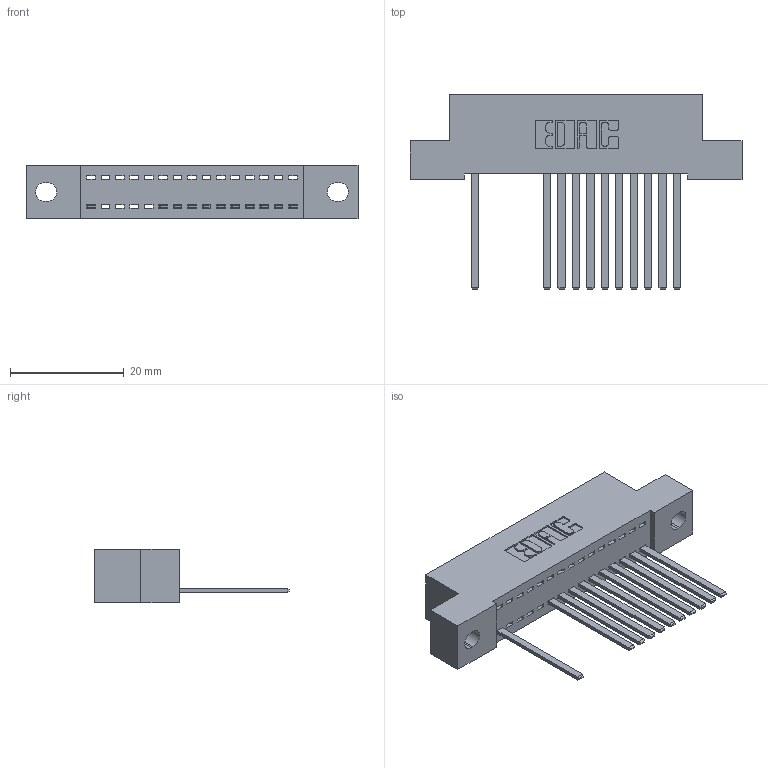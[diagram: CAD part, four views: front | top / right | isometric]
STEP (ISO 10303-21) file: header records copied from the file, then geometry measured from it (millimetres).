
FILE_DESCRIPTION (( 'STEP AP203' ), '1' );
FILE_NAME ('392-015-544-102.STEP', '2018-08-15T01:08:41', ( '' ), ( '' ), 'SwSTEP 2.0', 'SolidWorks 2016', '' );
FILE_SCHEMA (( 'CONFIG_CONTROL_DESIGN' ));
Length unit declared in the file: inch
Products named in the file (3): 342 Part_.128 Slot; 345-292-001_345-293-144; 392-015-544-102
Assembly tree (12 placements, depth 2):
  392-015-544-102
    342 Part_.128 Slot
    345-292-001_345-293-144  x11
Bounding box: 58.42 x 34.3 x 9.4 mm (x, y, z)
Volume: 5052.3 mm3; surface area: 6800.1 mm2
Topology: 12 solids, 12 shells, 734 faces, 2217 edges, 1462 vertices
Faces by surface type: plane 536, cylinder 198
Entity records: 12353 total; most frequent: CARTESIAN_POINT 2159, ORIENTED_EDGE 2114, DIRECTION 1867, EDGE_CURVE 1057, VECTOR 933, LINE 933, VERTEX_POINT 702, AXIS2_PLACEMENT_3D 467
